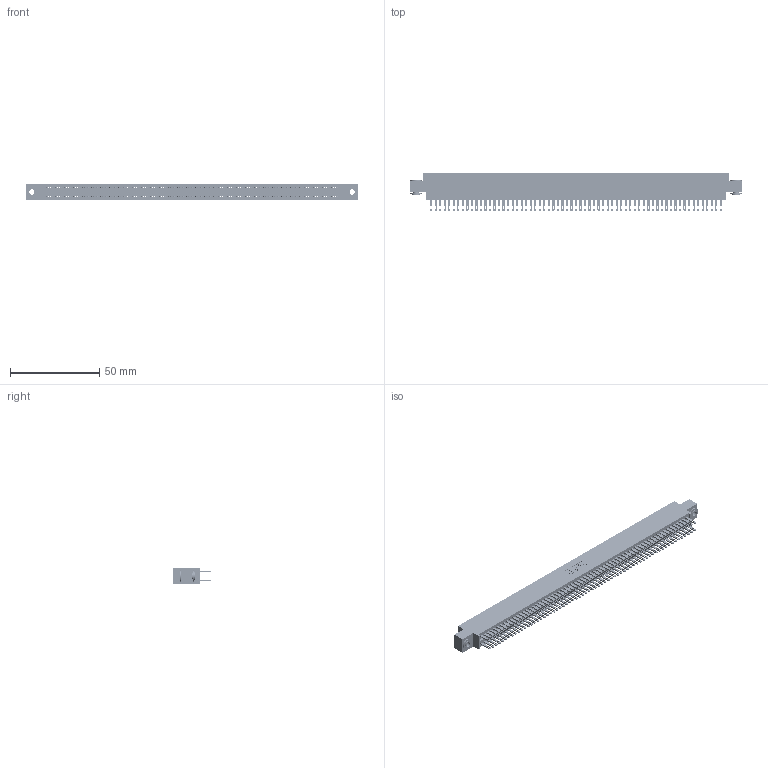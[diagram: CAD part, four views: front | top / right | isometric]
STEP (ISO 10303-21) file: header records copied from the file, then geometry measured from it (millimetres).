
FILE_DESCRIPTION (( 'STEP AP203' ), '1' );
FILE_NAME ('345-130-500-803.STEP', '2019-11-07T11:41:34', ( '' ), ( '' ), 'SwSTEP 2.0', 'SolidWorks 2016', '' );
FILE_SCHEMA (( 'CONFIG_CONTROL_DESIGN' ));
Length unit declared in the file: inch
Products named in the file (4): 345-292-001_345-293-100; 345-130-500-803; 345-250-002_345-250-002-102; 345 Part_0.170 Offset - 0.156 Dia-TH
Assembly tree (133 placements, depth 2):
  345-130-500-803
    345 Part_0.170 Offset - 0.156 Dia-TH
    345-292-001_345-293-100  x130
    345-250-002_345-250-002-102  x2
Bounding box: 186.31 x 21.51 x 9.4 mm (x, y, z)
Volume: 18615 mm3; surface area: 29635.9 mm2
Topology: 133 solids, 133 shells, 6148 faces, 18759 edges, 12502 vertices
Faces by surface type: plane 3604, cylinder 2536, cone 8
Entity records: 48616 total; most frequent: CARTESIAN_POINT 8103, ORIENTED_EDGE 8030, DIRECTION 7149, EDGE_CURVE 4015, VECTOR 3595, LINE 3595, VERTEX_POINT 2674, AXIS2_PLACEMENT_3D 1777
